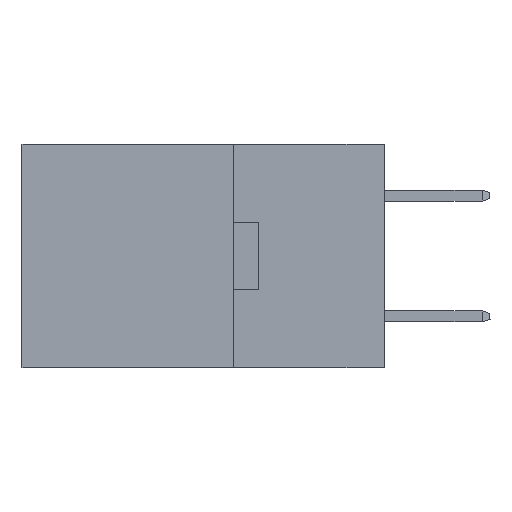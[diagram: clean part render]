
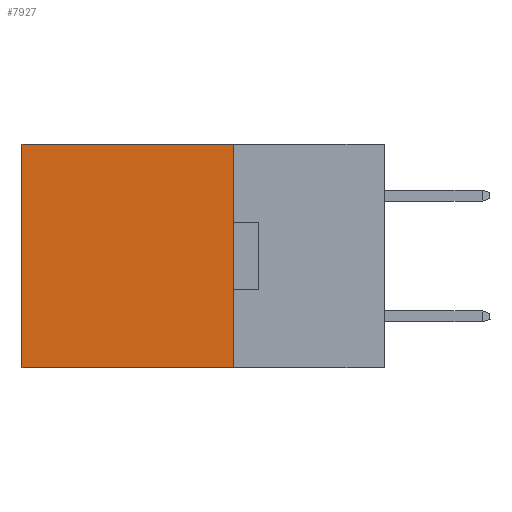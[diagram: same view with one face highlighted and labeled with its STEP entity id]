
A CAD part, left-side view. The second image highlights one B-rep face of the part: STEP entity #7927.
In plain terms, the highlighted planar face has unit normal (-1, 0, 0).
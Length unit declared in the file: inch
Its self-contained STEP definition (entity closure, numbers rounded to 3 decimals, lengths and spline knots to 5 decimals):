
#146 = CARTESIAN_POINT ( 'NONE',  ( 0.2615, 0.25, 0. ) ) ;
#236 = EDGE_CURVE ( 'NONE', #3307, #6407, #25003, .T. ) ;
#369 = CARTESIAN_POINT ( 'NONE',  ( 0.2615, 0.25, -0.37 ) ) ;
#611 = VECTOR ( 'NONE', #3145, 39.37008 ) ;
#1746 = ORIENTED_EDGE ( 'NONE', *, *, #21900, .F. ) ;
#2078 = CARTESIAN_POINT ( 'NONE',  ( 0.2615, 0.25, -0.37 ) ) ;
#2155 = CARTESIAN_POINT ( 'NONE',  ( 0.2615, 0.6, 0. ) ) ;
#2743 = DIRECTION ( 'NONE',  ( 1., 0., 0. ) ) ;
#3145 = DIRECTION ( 'NONE',  ( 0., 0., -1. ) ) ;
#3307 = VERTEX_POINT ( 'NONE', #146 ) ;
#3690 = DIRECTION ( 'NONE',  ( 0., 1., 0. ) ) ;
#3934 = DIRECTION ( 'NONE',  ( 0., 0., -1. ) ) ;
#4669 = FACE_OUTER_BOUND ( 'NONE', #15015, .T. ) ;
#6407 = VERTEX_POINT ( 'NONE', #2155 ) ;
#7867 = AXIS2_PLACEMENT_3D ( 'NONE', #9365, #2743, #18337 ) ;
#7918 = EDGE_CURVE ( 'NONE', #26950, #14203, #23131, .T. ) ;
#7927 = ADVANCED_FACE ( 'NONE', ( #4669 ), #16107, .F. ) ;
#9365 = CARTESIAN_POINT ( 'NONE',  ( 0.2615, 0.25, -0.37 ) ) ;
#10659 = LINE ( 'NONE', #15086, #22495 ) ;
#10800 = ORIENTED_EDGE ( 'NONE', *, *, #26646, .T. ) ;
#11186 = ORIENTED_EDGE ( 'NONE', *, *, #7918, .F. ) ;
#12490 = VECTOR ( 'NONE', #3690, 39.37008 ) ;
#14203 = VERTEX_POINT ( 'NONE', #21794 ) ;
#14845 = CARTESIAN_POINT ( 'NONE',  ( 0.2615, 0.25, 0. ) ) ;
#15015 = EDGE_LOOP ( 'NONE', ( #10800, #11186, #1746, #27856 ) ) ;
#15086 = CARTESIAN_POINT ( 'NONE',  ( 0.2615, 0.25, -0.37 ) ) ;
#16016 = DIRECTION ( 'NONE',  ( 0., 1., 0. ) ) ;
#16107 = PLANE ( 'NONE',  #7867 ) ;
#18337 = DIRECTION ( 'NONE',  ( 0., 0., -1. ) ) ;
#18737 = CARTESIAN_POINT ( 'NONE',  ( 0.2615, 0.6, -0.37 ) ) ;
#21794 = CARTESIAN_POINT ( 'NONE',  ( 0.2615, 0.6, -0.37 ) ) ;
#21900 = EDGE_CURVE ( 'NONE', #3307, #26950, #10659, .T. ) ;
#22447 = VECTOR ( 'NONE', #16016, 39.37008 ) ;
#22495 = VECTOR ( 'NONE', #3934, 39.37008 ) ;
#22930 = LINE ( 'NONE', #18737, #611 ) ;
#23131 = LINE ( 'NONE', #369, #22447 ) ;
#25003 = LINE ( 'NONE', #14845, #12490 ) ;
#26646 = EDGE_CURVE ( 'NONE', #6407, #14203, #22930, .T. ) ;
#26950 = VERTEX_POINT ( 'NONE', #2078 ) ;
#27856 = ORIENTED_EDGE ( 'NONE', *, *, #236, .T. ) ;
